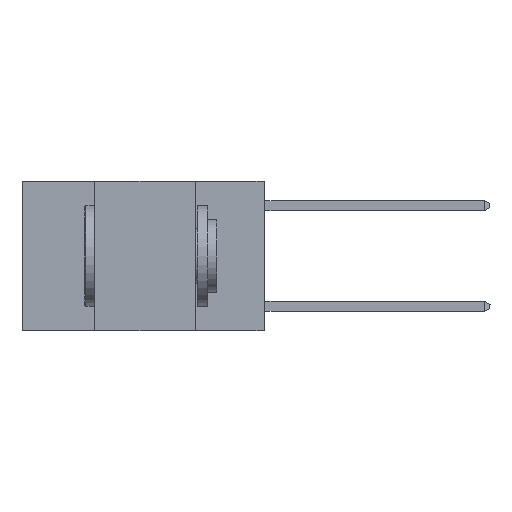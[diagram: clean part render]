
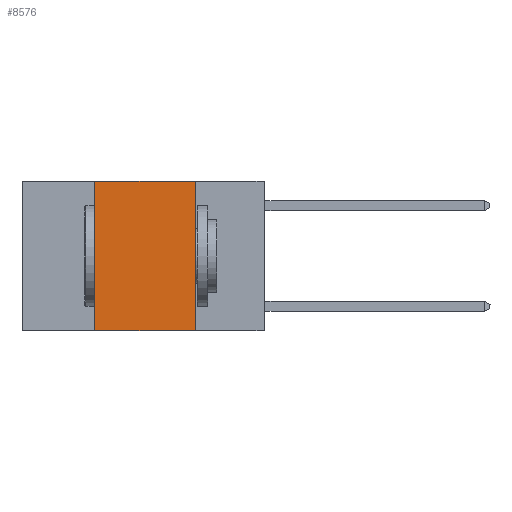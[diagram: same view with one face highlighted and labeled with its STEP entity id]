
A CAD part, left-side view. The second image highlights one B-rep face of the part: STEP entity #8576.
In plain terms, the highlighted planar face has unit normal (-1, 0, 0).
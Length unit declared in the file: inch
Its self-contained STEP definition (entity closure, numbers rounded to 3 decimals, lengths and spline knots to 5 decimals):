
#241 = PLANE ( 'NONE',  #8330 ) ;
#871 = VERTEX_POINT ( 'NONE', #1628 ) ;
#1018 = DIRECTION ( 'NONE',  ( 1., 0., 0. ) ) ;
#1304 = VERTEX_POINT ( 'NONE', #2447 ) ;
#1628 = CARTESIAN_POINT ( 'NONE',  ( 0., 0.17, -0.37 ) ) ;
#1660 = DIRECTION ( 'NONE',  ( 0., -1., 0. ) ) ;
#1694 = CARTESIAN_POINT ( 'NONE',  ( 0., 0.6, -0.37 ) ) ;
#2314 = FACE_OUTER_BOUND ( 'NONE', #6189, .T. ) ;
#2447 = CARTESIAN_POINT ( 'NONE',  ( 0., 0.17, 0. ) ) ;
#3454 = DIRECTION ( 'NONE',  ( 0., -1., 0. ) ) ;
#3625 = VECTOR ( 'NONE', #6849, 39.37008 ) ;
#3742 = VECTOR ( 'NONE', #8742, 39.37008 ) ;
#3747 = ORIENTED_EDGE ( 'NONE', *, *, #8182, .F. ) ;
#3793 = ORIENTED_EDGE ( 'NONE', *, *, #7948, .F. ) ;
#3831 = EDGE_CURVE ( 'NONE', #8201, #871, #6419, .T. ) ;
#4407 = LINE ( 'NONE', #8553, #8053 ) ;
#5424 = CARTESIAN_POINT ( 'NONE',  ( 0., 0.42, -0.37 ) ) ;
#5554 = VERTEX_POINT ( 'NONE', #6116 ) ;
#5574 = CARTESIAN_POINT ( 'NONE',  ( 0., 0.6, 0. ) ) ;
#5868 = EDGE_CURVE ( 'NONE', #5554, #1304, #4407, .T. ) ;
#5990 = VECTOR ( 'NONE', #1660, 39.37008 ) ;
#6116 = CARTESIAN_POINT ( 'NONE',  ( 0., 0.42, 0. ) ) ;
#6131 = CARTESIAN_POINT ( 'NONE',  ( 0., 0.42, 0. ) ) ;
#6189 = EDGE_LOOP ( 'NONE', ( #3793, #8394, #3747, #9343 ) ) ;
#6286 = DIRECTION ( 'NONE',  ( 0., 0., -1. ) ) ;
#6419 = LINE ( 'NONE', #1694, #5990 ) ;
#6849 = DIRECTION ( 'NONE',  ( 0., 0., 1. ) ) ;
#7642 = LINE ( 'NONE', #8026, #3742 ) ;
#7948 = EDGE_CURVE ( 'NONE', #1304, #871, #7642, .T. ) ;
#8026 = CARTESIAN_POINT ( 'NONE',  ( 0., 0.17, 0. ) ) ;
#8053 = VECTOR ( 'NONE', #3454, 39.37008 ) ;
#8182 = EDGE_CURVE ( 'NONE', #8201, #5554, #9401, .T. ) ;
#8201 = VERTEX_POINT ( 'NONE', #5424 ) ;
#8330 = AXIS2_PLACEMENT_3D ( 'NONE', #5574, #1018, #6286 ) ;
#8394 = ORIENTED_EDGE ( 'NONE', *, *, #5868, .F. ) ;
#8553 = CARTESIAN_POINT ( 'NONE',  ( 0., 0.6, 0. ) ) ;
#8576 = ADVANCED_FACE ( 'NONE', ( #2314 ), #241, .F. ) ;
#8742 = DIRECTION ( 'NONE',  ( 0., 0., -1. ) ) ;
#9343 = ORIENTED_EDGE ( 'NONE', *, *, #3831, .T. ) ;
#9401 = LINE ( 'NONE', #6131, #3625 ) ;
